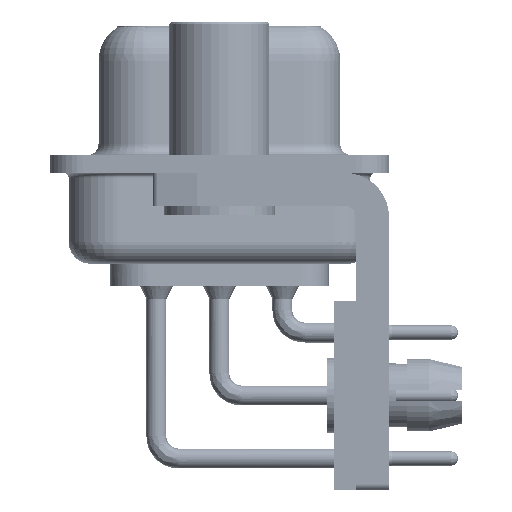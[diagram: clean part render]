
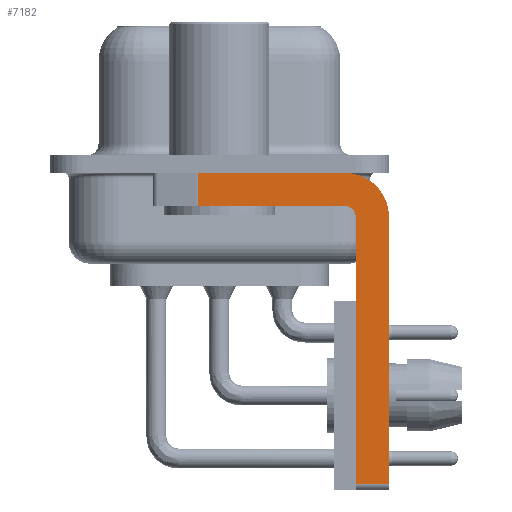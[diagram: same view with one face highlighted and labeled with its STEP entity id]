
A CAD part, left-side view. The second image highlights one B-rep face of the part: STEP entity #7182.
In plain terms, the highlighted planar face has unit normal (-1, 0, 0).
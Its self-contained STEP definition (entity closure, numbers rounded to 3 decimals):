
#475 = CARTESIAN_POINT ( 'NONE',  ( -2.9, -5.65, -1.9 ) ) ;
#859 = CARTESIAN_POINT ( 'NONE',  ( -2.9, -5.65, -0.4 ) ) ;
#974 = CARTESIAN_POINT ( 'NONE',  ( -2.9, -6.15, -2.4 ) ) ;
#1508 = EDGE_CURVE ( 'NONE', #3866, #21229, #12018, .T. ) ;
#1852 = ORIENTED_EDGE ( 'NONE', *, *, #27619, .T. ) ;
#2182 = CIRCLE ( 'NONE', #29416, 0.5 ) ;
#2738 = CARTESIAN_POINT ( 'NONE',  ( -2.9, -5.65, -14.45 ) ) ;
#3562 = VECTOR ( 'NONE', #8241, 1000. ) ;
#3866 = VERTEX_POINT ( 'NONE', #33757 ) ;
#4890 = ORIENTED_EDGE ( 'NONE', *, *, #1508, .F. ) ;
#6294 = DIRECTION ( 'NONE',  ( 1., 0., 0. ) ) ;
#6949 = AXIS2_PLACEMENT_3D ( 'NONE', #34613, #6294, #28507 ) ;
#7182 = ADVANCED_FACE ( 'NONE', ( #28969 ), #37786, .F. ) ;
#7982 = EDGE_LOOP ( 'NONE', ( #40475, #19677, #17043, #36020, #38977, #1852, #4890, #37771 ) ) ;
#8114 = EDGE_CURVE ( 'NONE', #32351, #3866, #23462, .T. ) ;
#8241 = DIRECTION ( 'NONE',  ( 0., 0., -1. ) ) ;
#8308 = DIRECTION ( 'NONE',  ( -1., 0., 0. ) ) ;
#8854 = VECTOR ( 'NONE', #30457, 1000. ) ;
#9244 = CARTESIAN_POINT ( 'NONE',  ( -2.9, 0.978, -1.9 ) ) ;
#9421 = CARTESIAN_POINT ( 'NONE',  ( -2.9, -7.65, -14.45 ) ) ;
#9652 = VECTOR ( 'NONE', #21490, 1000. ) ;
#9827 = LINE ( 'NONE', #11518, #8854 ) ;
#10453 = CARTESIAN_POINT ( 'NONE',  ( -2.9, -6.15, -14.45 ) ) ;
#11180 = CARTESIAN_POINT ( 'NONE',  ( -2.9, 0.978, -0.4 ) ) ;
#11518 = CARTESIAN_POINT ( 'NONE',  ( -2.9, -6.15, -14.7 ) ) ;
#11886 = VECTOR ( 'NONE', #21738, 1000. ) ;
#12018 = LINE ( 'NONE', #29080, #3562 ) ;
#12250 = EDGE_CURVE ( 'NONE', #21042, #30360, #34806, .T. ) ;
#13047 = VERTEX_POINT ( 'NONE', #11180 ) ;
#14026 = DIRECTION ( 'NONE',  ( 1., 0., 0. ) ) ;
#15183 = VECTOR ( 'NONE', #24208, 1000. ) ;
#16791 = EDGE_CURVE ( 'NONE', #23145, #21042, #2182, .T. ) ;
#17043 = ORIENTED_EDGE ( 'NONE', *, *, #12250, .F. ) ;
#19677 = ORIENTED_EDGE ( 'NONE', *, *, #36747, .T. ) ;
#20348 = VECTOR ( 'NONE', #31372, 1000. ) ;
#20666 = LINE ( 'NONE', #24343, #15183 ) ;
#21042 = VERTEX_POINT ( 'NONE', #475 ) ;
#21229 = VERTEX_POINT ( 'NONE', #9421 ) ;
#21490 = DIRECTION ( 'NONE',  ( 0., 1., 0. ) ) ;
#21738 = DIRECTION ( 'NONE',  ( 0., -1., 0. ) ) ;
#22734 = EDGE_CURVE ( 'NONE', #13047, #32351, #20666, .T. ) ;
#23145 = VERTEX_POINT ( 'NONE', #974 ) ;
#23462 = CIRCLE ( 'NONE', #36360, 2. ) ;
#24208 = DIRECTION ( 'NONE',  ( 0., -1., 0. ) ) ;
#24343 = CARTESIAN_POINT ( 'NONE',  ( -2.9, 3., -0.4 ) ) ;
#24710 = CARTESIAN_POINT ( 'NONE',  ( -2.9, -5.65, -1.9 ) ) ;
#27351 = CARTESIAN_POINT ( 'NONE',  ( -2.9, -5.65, -2.4 ) ) ;
#27619 = EDGE_CURVE ( 'NONE', #36110, #21229, #28748, .T. ) ;
#28507 = DIRECTION ( 'NONE',  ( 0., 0., -1. ) ) ;
#28748 = LINE ( 'NONE', #2738, #11886 ) ;
#28969 = FACE_OUTER_BOUND ( 'NONE', #7982, .T. ) ;
#29080 = CARTESIAN_POINT ( 'NONE',  ( -2.9, -7.65, -2.4 ) ) ;
#29416 = AXIS2_PLACEMENT_3D ( 'NONE', #27351, #8308, #30460 ) ;
#29482 = CARTESIAN_POINT ( 'NONE',  ( -2.9, 0.978, -1.9 ) ) ;
#30360 = VERTEX_POINT ( 'NONE', #29482 ) ;
#30457 = DIRECTION ( 'NONE',  ( 0., 0., 1. ) ) ;
#30460 = DIRECTION ( 'NONE',  ( 0., 0., 1. ) ) ;
#31372 = DIRECTION ( 'NONE',  ( 0., 0., -1. ) ) ;
#32351 = VERTEX_POINT ( 'NONE', #859 ) ;
#32613 = EDGE_CURVE ( 'NONE', #36110, #23145, #9827, .T. ) ;
#32963 = CARTESIAN_POINT ( 'NONE',  ( -2.9, -5.65, -2.4 ) ) ;
#33757 = CARTESIAN_POINT ( 'NONE',  ( -2.9, -7.65, -2.4 ) ) ;
#34613 = CARTESIAN_POINT ( 'NONE',  ( -2.9, -5.65, -2.4 ) ) ;
#34806 = LINE ( 'NONE', #24710, #9652 ) ;
#36020 = ORIENTED_EDGE ( 'NONE', *, *, #16791, .F. ) ;
#36081 = DIRECTION ( 'NONE',  ( 0., 0., -1. ) ) ;
#36110 = VERTEX_POINT ( 'NONE', #10453 ) ;
#36360 = AXIS2_PLACEMENT_3D ( 'NONE', #32963, #14026, #36081 ) ;
#36747 = EDGE_CURVE ( 'NONE', #13047, #30360, #38034, .T. ) ;
#37771 = ORIENTED_EDGE ( 'NONE', *, *, #8114, .F. ) ;
#37786 = PLANE ( 'NONE',  #6949 ) ;
#38034 = LINE ( 'NONE', #9244, #20348 ) ;
#38977 = ORIENTED_EDGE ( 'NONE', *, *, #32613, .F. ) ;
#40475 = ORIENTED_EDGE ( 'NONE', *, *, #22734, .F. ) ;
